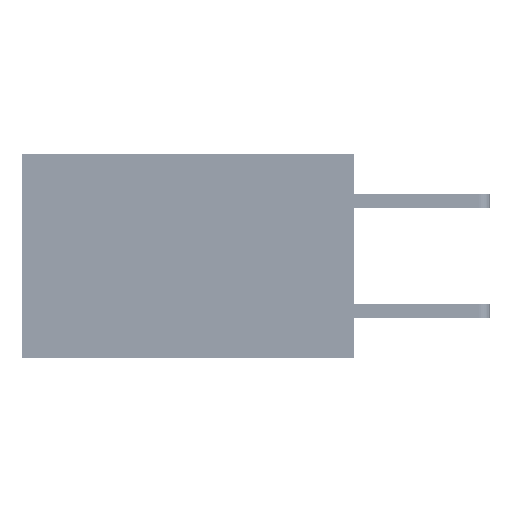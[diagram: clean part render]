
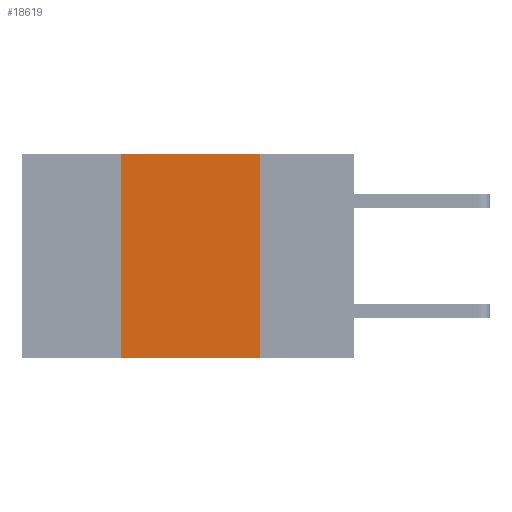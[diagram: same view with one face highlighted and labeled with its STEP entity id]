
A CAD part, left-side view. The second image highlights one B-rep face of the part: STEP entity #18619.
In plain terms, the highlighted planar face has unit normal (-1, 0, 0).
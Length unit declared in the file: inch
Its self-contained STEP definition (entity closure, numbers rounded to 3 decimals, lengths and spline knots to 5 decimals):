
#5059 = LINE ( 'NONE', #18716, #10783 ) ;
#5289 = VERTEX_POINT ( 'NONE', #13666 ) ;
#5362 = VECTOR ( 'NONE', #22432, 39.37008 ) ;
#5538 = CARTESIAN_POINT ( 'NONE',  ( 0., 0.6, 0. ) ) ;
#5644 = EDGE_LOOP ( 'NONE', ( #37709, #25034, #14181, #28512 ) ) ;
#5780 = CARTESIAN_POINT ( 'NONE',  ( 0., 0.17, -0.37 ) ) ;
#6671 = LINE ( 'NONE', #22533, #10973 ) ;
#10136 = DIRECTION ( 'NONE',  ( 0., 0., 1. ) ) ;
#10166 = VERTEX_POINT ( 'NONE', #5780 ) ;
#10783 = VECTOR ( 'NONE', #25323, 39.37008 ) ;
#10816 = CARTESIAN_POINT ( 'NONE',  ( 0., 0.6, -0.37 ) ) ;
#10973 = VECTOR ( 'NONE', #10136, 39.37008 ) ;
#11356 = FACE_OUTER_BOUND ( 'NONE', #5644, .T. ) ;
#12662 = EDGE_CURVE ( 'NONE', #5289, #10166, #27799, .T. ) ;
#12858 = VERTEX_POINT ( 'NONE', #28172 ) ;
#13666 = CARTESIAN_POINT ( 'NONE',  ( 0., 0.17, 0. ) ) ;
#14180 = LINE ( 'NONE', #10816, #35169 ) ;
#14181 = ORIENTED_EDGE ( 'NONE', *, *, #37656, .F. ) ;
#17475 = VERTEX_POINT ( 'NONE', #19309 ) ;
#18514 = CARTESIAN_POINT ( 'NONE',  ( 0., 0.17, 0. ) ) ;
#18619 = ADVANCED_FACE ( 'NONE', ( #11356 ), #26671, .F. ) ;
#18716 = CARTESIAN_POINT ( 'NONE',  ( 0., 0.6, 0. ) ) ;
#19309 = CARTESIAN_POINT ( 'NONE',  ( 0., 0.42, 0. ) ) ;
#19453 = EDGE_CURVE ( 'NONE', #17475, #5289, #5059, .T. ) ;
#22432 = DIRECTION ( 'NONE',  ( 0., 0., -1. ) ) ;
#22533 = CARTESIAN_POINT ( 'NONE',  ( 0., 0.42, 0. ) ) ;
#23228 = DIRECTION ( 'NONE',  ( 0., -1., 0. ) ) ;
#25034 = ORIENTED_EDGE ( 'NONE', *, *, #19453, .F. ) ;
#25323 = DIRECTION ( 'NONE',  ( 0., -1., 0. ) ) ;
#25821 = AXIS2_PLACEMENT_3D ( 'NONE', #5538, #26791, #36197 ) ;
#26671 = PLANE ( 'NONE',  #25821 ) ;
#26791 = DIRECTION ( 'NONE',  ( 1., 0., 0. ) ) ;
#27799 = LINE ( 'NONE', #18514, #5362 ) ;
#28172 = CARTESIAN_POINT ( 'NONE',  ( 0., 0.42, -0.37 ) ) ;
#28512 = ORIENTED_EDGE ( 'NONE', *, *, #33259, .T. ) ;
#33259 = EDGE_CURVE ( 'NONE', #12858, #10166, #14180, .T. ) ;
#35169 = VECTOR ( 'NONE', #23228, 39.37008 ) ;
#36197 = DIRECTION ( 'NONE',  ( 0., 0., -1. ) ) ;
#37656 = EDGE_CURVE ( 'NONE', #12858, #17475, #6671, .T. ) ;
#37709 = ORIENTED_EDGE ( 'NONE', *, *, #12662, .F. ) ;
